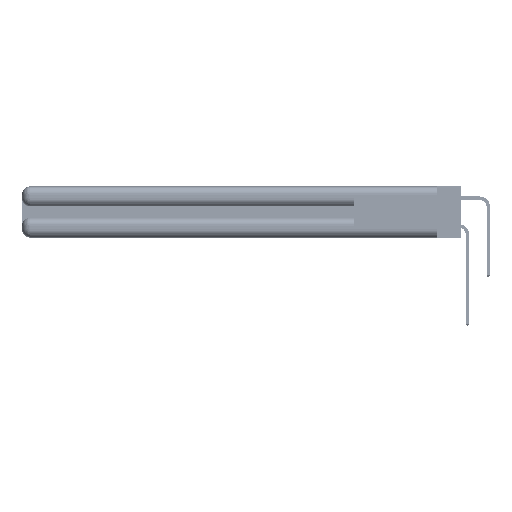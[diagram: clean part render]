
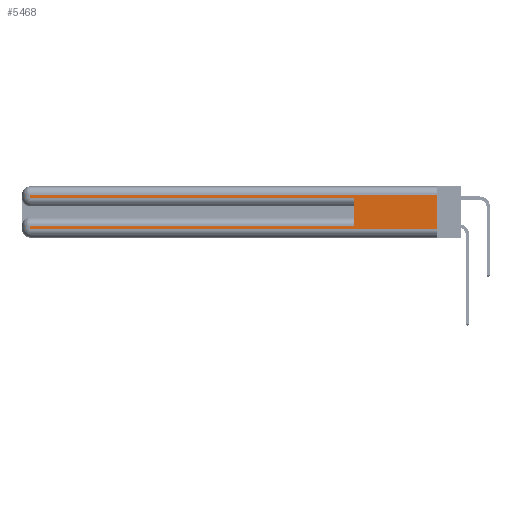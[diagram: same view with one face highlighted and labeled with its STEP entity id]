
A CAD part, left-side view. The second image highlights one B-rep face of the part: STEP entity #5468.
In plain terms, the highlighted planar face has unit normal (-1, 0, 0).
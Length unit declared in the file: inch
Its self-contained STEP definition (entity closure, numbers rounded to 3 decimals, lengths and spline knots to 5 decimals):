
#372 = DIRECTION ( 'NONE',  ( 0., 0., -1. ) ) ;
#1336 = DIRECTION ( 'NONE',  ( 0., 0., -1. ) ) ;
#1468 = AXIS2_PLACEMENT_3D ( 'NONE', #32239, #24409, #372 ) ;
#2056 = CARTESIAN_POINT ( 'NONE',  ( 0., 0., 0.285 ) ) ;
#2074 = VERTEX_POINT ( 'NONE', #27116 ) ;
#2393 = EDGE_CURVE ( 'NONE', #33673, #2074, #35136, .T. ) ;
#3252 = EDGE_CURVE ( 'NONE', #25568, #2074, #50523, .T. ) ;
#5348 = LINE ( 'NONE', #40419, #17273 ) ;
#5468 = ADVANCED_FACE ( 'NONE', ( #23564 ), #8295, .F. ) ;
#7072 = VECTOR ( 'NONE', #1336, 39.37008 ) ;
#8295 = PLANE ( 'NONE',  #1468 ) ;
#10236 = VERTEX_POINT ( 'NONE', #36775 ) ;
#12347 = VERTEX_POINT ( 'NONE', #23027 ) ;
#13095 = VERTEX_POINT ( 'NONE', #23836 ) ;
#13861 = VECTOR ( 'NONE', #45057, 39.37008 ) ;
#14131 = CARTESIAN_POINT ( 'NONE',  ( 0., 2.94, 0.37 ) ) ;
#16395 = VERTEX_POINT ( 'NONE', #19577 ) ;
#16405 = EDGE_CURVE ( 'NONE', #12347, #13095, #43994, .T. ) ;
#16704 = ORIENTED_EDGE ( 'NONE', *, *, #50079, .T. ) ;
#16835 = CARTESIAN_POINT ( 'NONE',  ( 0., 0., 0.31 ) ) ;
#17273 = VECTOR ( 'NONE', #44418, 39.37008 ) ;
#17452 = CARTESIAN_POINT ( 'NONE',  ( 0., 0., 0.31 ) ) ;
#18295 = EDGE_CURVE ( 'NONE', #10236, #13095, #50580, .T. ) ;
#18822 = VECTOR ( 'NONE', #26086, 39.37008 ) ;
#19577 = CARTESIAN_POINT ( 'NONE',  ( 0., 2.94, 0.085 ) ) ;
#20257 = LINE ( 'NONE', #49146, #7072 ) ;
#20600 = CARTESIAN_POINT ( 'NONE',  ( 0., 2.94, 0.06 ) ) ;
#21625 = ORIENTED_EDGE ( 'NONE', *, *, #2393, .F. ) ;
#22518 = EDGE_CURVE ( 'NONE', #12347, #16395, #5348, .T. ) ;
#23027 = CARTESIAN_POINT ( 'NONE',  ( 0., 0.6, 0.085 ) ) ;
#23036 = VERTEX_POINT ( 'NONE', #51416 ) ;
#23366 = LINE ( 'NONE', #14131, #35260 ) ;
#23564 = FACE_OUTER_BOUND ( 'NONE', #48107, .T. ) ;
#23836 = CARTESIAN_POINT ( 'NONE',  ( 0., 0.6, 0.285 ) ) ;
#24216 = ORIENTED_EDGE ( 'NONE', *, *, #16405, .F. ) ;
#24409 = DIRECTION ( 'NONE',  ( 1., 0., 0. ) ) ;
#25568 = VERTEX_POINT ( 'NONE', #20600 ) ;
#26086 = DIRECTION ( 'NONE',  ( 0., -1., 0. ) ) ;
#27116 = CARTESIAN_POINT ( 'NONE',  ( 0., 0., 0.06 ) ) ;
#31621 = DIRECTION ( 'NONE',  ( 0., 0., 1. ) ) ;
#32175 = VECTOR ( 'NONE', #31621, 39.37008 ) ;
#32239 = CARTESIAN_POINT ( 'NONE',  ( 0., 0., 0.37 ) ) ;
#32986 = ORIENTED_EDGE ( 'NONE', *, *, #18295, .T. ) ;
#33673 = VERTEX_POINT ( 'NONE', #16835 ) ;
#33836 = CARTESIAN_POINT ( 'NONE',  ( 0., 0., 0.06 ) ) ;
#33891 = ORIENTED_EDGE ( 'NONE', *, *, #22518, .T. ) ;
#34390 = EDGE_CURVE ( 'NONE', #33673, #23036, #46604, .T. ) ;
#35136 = LINE ( 'NONE', #41048, #13861 ) ;
#35260 = VECTOR ( 'NONE', #46030, 39.37008 ) ;
#36775 = CARTESIAN_POINT ( 'NONE',  ( 0., 2.94, 0.285 ) ) ;
#37371 = DIRECTION ( 'NONE',  ( 0., 1., 0. ) ) ;
#38029 = DIRECTION ( 'NONE',  ( 0., -1., 0. ) ) ;
#38712 = ORIENTED_EDGE ( 'NONE', *, *, #3252, .T. ) ;
#38798 = VECTOR ( 'NONE', #38029, 39.37008 ) ;
#40419 = CARTESIAN_POINT ( 'NONE',  ( 0., 0., 0.085 ) ) ;
#40585 = ORIENTED_EDGE ( 'NONE', *, *, #34390, .T. ) ;
#41048 = CARTESIAN_POINT ( 'NONE',  ( 0., 0., 0.37 ) ) ;
#41610 = VECTOR ( 'NONE', #37371, 39.37008 ) ;
#43459 = CARTESIAN_POINT ( 'NONE',  ( 0., 0.6, 0.145 ) ) ;
#43994 = LINE ( 'NONE', #43459, #32175 ) ;
#44418 = DIRECTION ( 'NONE',  ( 0., 1., 0. ) ) ;
#45057 = DIRECTION ( 'NONE',  ( 0., 0., -1. ) ) ;
#46030 = DIRECTION ( 'NONE',  ( 0., 0., -1. ) ) ;
#46604 = LINE ( 'NONE', #17452, #41610 ) ;
#47700 = ORIENTED_EDGE ( 'NONE', *, *, #49934, .T. ) ;
#48107 = EDGE_LOOP ( 'NONE', ( #21625, #40585, #16704, #32986, #24216, #33891, #47700, #38712 ) ) ;
#49146 = CARTESIAN_POINT ( 'NONE',  ( 0., 2.94, 0.37 ) ) ;
#49934 = EDGE_CURVE ( 'NONE', #16395, #25568, #20257, .T. ) ;
#50079 = EDGE_CURVE ( 'NONE', #23036, #10236, #23366, .T. ) ;
#50523 = LINE ( 'NONE', #33836, #38798 ) ;
#50580 = LINE ( 'NONE', #2056, #18822 ) ;
#51416 = CARTESIAN_POINT ( 'NONE',  ( 0., 2.94, 0.31 ) ) ;
